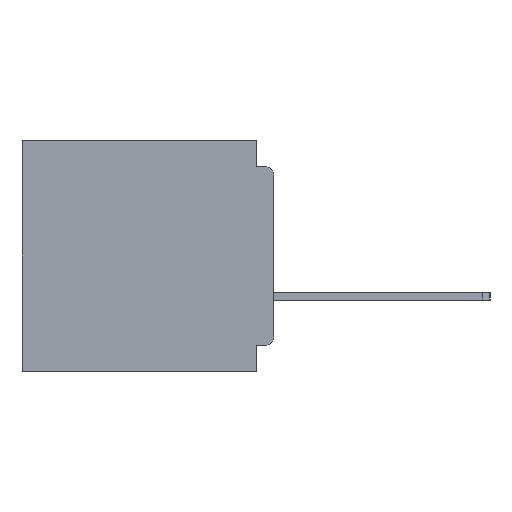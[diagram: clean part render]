
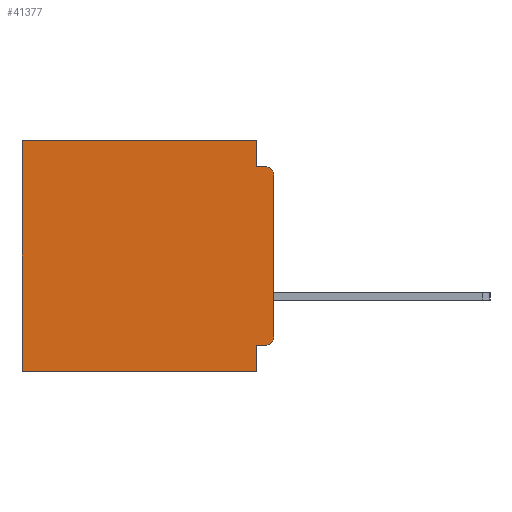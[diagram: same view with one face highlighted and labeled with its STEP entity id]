
A CAD part, left-side view. The second image highlights one B-rep face of the part: STEP entity #41377.
In plain terms, the highlighted planar face has unit normal (-1, 0, 0).
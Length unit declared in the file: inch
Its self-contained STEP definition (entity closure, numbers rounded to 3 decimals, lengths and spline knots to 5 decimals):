
#357 = AXIS2_PLACEMENT_3D ( 'NONE', #12856, #17834, #52186 ) ;
#528 = EDGE_CURVE ( 'NONE', #32303, #37660, #52629, .T. ) ;
#1546 = DIRECTION ( 'NONE',  ( 0., 0., -1. ) ) ;
#2589 = DIRECTION ( 'NONE',  ( 0., 1., 0. ) ) ;
#4182 = VERTEX_POINT ( 'NONE', #36759 ) ;
#5727 = CARTESIAN_POINT ( 'NONE',  ( 0.3, 0.437, 0. ) ) ;
#5845 = LINE ( 'NONE', #41670, #58177 ) ;
#7644 = DIRECTION ( 'NONE',  ( 0., -1., 0. ) ) ;
#7784 = DIRECTION ( 'NONE',  ( 0., 0., -1. ) ) ;
#7849 = PLANE ( 'NONE',  #357 ) ;
#8035 = LINE ( 'NONE', #10522, #58827 ) ;
#9507 = VECTOR ( 'NONE', #7784, 39.37008 ) ;
#10188 = ORIENTED_EDGE ( 'NONE', *, *, #16165, .F. ) ;
#10325 = CARTESIAN_POINT ( 'NONE',  ( 0.3, 0.437, -0.4 ) ) ;
#10521 = CARTESIAN_POINT ( 'NONE',  ( 0.3, 0.031, -0.4 ) ) ;
#10522 = CARTESIAN_POINT ( 'NONE',  ( 0.3, 0., -0.4 ) ) ;
#10952 = EDGE_CURVE ( 'NONE', #42358, #20097, #8035, .T. ) ;
#12225 = DIRECTION ( 'NONE',  ( 0., 0., -1. ) ) ;
#12282 = VECTOR ( 'NONE', #7644, 39.37008 ) ;
#12856 = CARTESIAN_POINT ( 'NONE',  ( 0.3, 0., -0.4 ) ) ;
#14637 = EDGE_CURVE ( 'NONE', #51846, #29714, #25428, .T. ) ;
#15506 = DIRECTION ( 'NONE',  ( 0., 1., 0. ) ) ;
#16084 = CARTESIAN_POINT ( 'NONE',  ( 0.3, 0.015, -0.355 ) ) ;
#16165 = EDGE_CURVE ( 'NONE', #32303, #4182, #53643, .T. ) ;
#16231 = VECTOR ( 'NONE', #40010, 39.37008 ) ;
#16594 = VECTOR ( 'NONE', #47403, 39.37008 ) ;
#17834 = DIRECTION ( 'NONE',  ( 1., 0., 0. ) ) ;
#17983 = CARTESIAN_POINT ( 'NONE',  ( 0.3, 0., -0.4 ) ) ;
#20070 = CARTESIAN_POINT ( 'NONE',  ( 0.3, 0., -0.34 ) ) ;
#20097 = VERTEX_POINT ( 'NONE', #10325 ) ;
#20775 = DIRECTION ( 'NONE',  ( 0., 0., -1. ) ) ;
#23938 = CARTESIAN_POINT ( 'NONE',  ( 0.3, 0., -0.355 ) ) ;
#24062 = ORIENTED_EDGE ( 'NONE', *, *, #52213, .F. ) ;
#24577 = CARTESIAN_POINT ( 'NONE',  ( 0.3, 0.031, 0. ) ) ;
#25428 = LINE ( 'NONE', #41870, #12282 ) ;
#26673 = ORIENTED_EDGE ( 'NONE', *, *, #38209, .F. ) ;
#27033 = EDGE_LOOP ( 'NONE', ( #24062, #42827, #41195, #38674, #60316, #49272, #55585, #26673, #10188, #35928 ) ) ;
#28915 = DIRECTION ( 'NONE',  ( 0., 1., 0. ) ) ;
#29714 = VERTEX_POINT ( 'NONE', #36607 ) ;
#31206 = DIRECTION ( 'NONE',  ( -1., 0., 0. ) ) ;
#31578 = CIRCLE ( 'NONE', #54038, 0.015 ) ;
#32303 = VERTEX_POINT ( 'NONE', #16084 ) ;
#34575 = VECTOR ( 'NONE', #2589, 39.37008 ) ;
#34629 = VERTEX_POINT ( 'NONE', #24577 ) ;
#34934 = EDGE_CURVE ( 'NONE', #38225, #20097, #5845, .T. ) ;
#35928 = ORIENTED_EDGE ( 'NONE', *, *, #528, .T. ) ;
#36130 = LINE ( 'NONE', #42026, #34575 ) ;
#36607 = CARTESIAN_POINT ( 'NONE',  ( 0.3, 0.015, -0.045 ) ) ;
#36759 = CARTESIAN_POINT ( 'NONE',  ( 0.3, 0.031, -0.355 ) ) ;
#37660 = VERTEX_POINT ( 'NONE', #20070 ) ;
#38209 = EDGE_CURVE ( 'NONE', #4182, #42358, #55412, .T. ) ;
#38225 = VERTEX_POINT ( 'NONE', #5727 ) ;
#38674 = ORIENTED_EDGE ( 'NONE', *, *, #43709, .F. ) ;
#39040 = VECTOR ( 'NONE', #28915, 39.37008 ) ;
#39829 = EDGE_CURVE ( 'NONE', #34629, #38225, #36130, .T. ) ;
#40010 = DIRECTION ( 'NONE',  ( 0., 0., -1. ) ) ;
#40821 = CARTESIAN_POINT ( 'NONE',  ( 0.3, 0., -0.06 ) ) ;
#41195 = ORIENTED_EDGE ( 'NONE', *, *, #14637, .F. ) ;
#41201 = AXIS2_PLACEMENT_3D ( 'NONE', #46380, #46174, #20775 ) ;
#41377 = ADVANCED_FACE ( 'NONE', ( #43523 ), #7849, .F. ) ;
#41670 = CARTESIAN_POINT ( 'NONE',  ( 0.3, 0.437, -0.4 ) ) ;
#41870 = CARTESIAN_POINT ( 'NONE',  ( 0.3, 0., -0.045 ) ) ;
#42026 = CARTESIAN_POINT ( 'NONE',  ( 0.3, 0., 0. ) ) ;
#42358 = VERTEX_POINT ( 'NONE', #55935 ) ;
#42827 = ORIENTED_EDGE ( 'NONE', *, *, #49662, .T. ) ;
#43523 = FACE_OUTER_BOUND ( 'NONE', #27033, .T. ) ;
#43709 = EDGE_CURVE ( 'NONE', #34629, #51846, #48803, .T. ) ;
#46174 = DIRECTION ( 'NONE',  ( -1., 0., 0. ) ) ;
#46380 = CARTESIAN_POINT ( 'NONE',  ( 0.3, 0.015, -0.34 ) ) ;
#47403 = DIRECTION ( 'NONE',  ( 0., 0., -1. ) ) ;
#48803 = LINE ( 'NONE', #56853, #9507 ) ;
#49272 = ORIENTED_EDGE ( 'NONE', *, *, #34934, .T. ) ;
#49662 = EDGE_CURVE ( 'NONE', #49686, #29714, #31578, .T. ) ;
#49686 = VERTEX_POINT ( 'NONE', #40821 ) ;
#51846 = VERTEX_POINT ( 'NONE', #58344 ) ;
#52186 = DIRECTION ( 'NONE',  ( 0., 0., -1. ) ) ;
#52213 = EDGE_CURVE ( 'NONE', #49686, #37660, #55761, .T. ) ;
#52629 = CIRCLE ( 'NONE', #41201, 0.015 ) ;
#53643 = LINE ( 'NONE', #23938, #39040 ) ;
#54038 = AXIS2_PLACEMENT_3D ( 'NONE', #60524, #31206, #1546 ) ;
#55412 = LINE ( 'NONE', #10521, #16231 ) ;
#55585 = ORIENTED_EDGE ( 'NONE', *, *, #10952, .F. ) ;
#55761 = LINE ( 'NONE', #17983, #16594 ) ;
#55935 = CARTESIAN_POINT ( 'NONE',  ( 0.3, 0.031, -0.4 ) ) ;
#56853 = CARTESIAN_POINT ( 'NONE',  ( 0.3, 0.031, 0. ) ) ;
#58177 = VECTOR ( 'NONE', #12225, 39.37008 ) ;
#58344 = CARTESIAN_POINT ( 'NONE',  ( 0.3, 0.031, -0.045 ) ) ;
#58827 = VECTOR ( 'NONE', #15506, 39.37008 ) ;
#60316 = ORIENTED_EDGE ( 'NONE', *, *, #39829, .T. ) ;
#60524 = CARTESIAN_POINT ( 'NONE',  ( 0.3, 0.015, -0.06 ) ) ;
